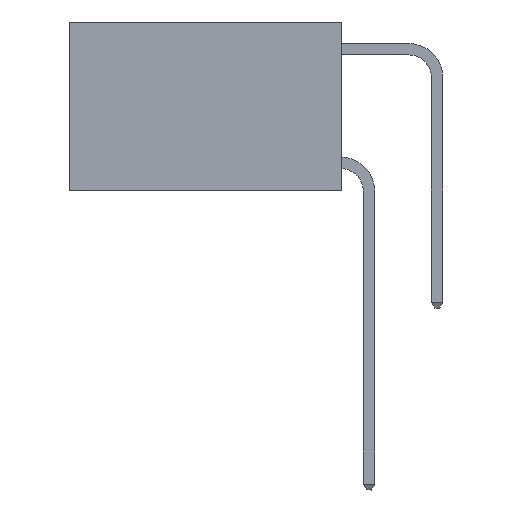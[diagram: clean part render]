
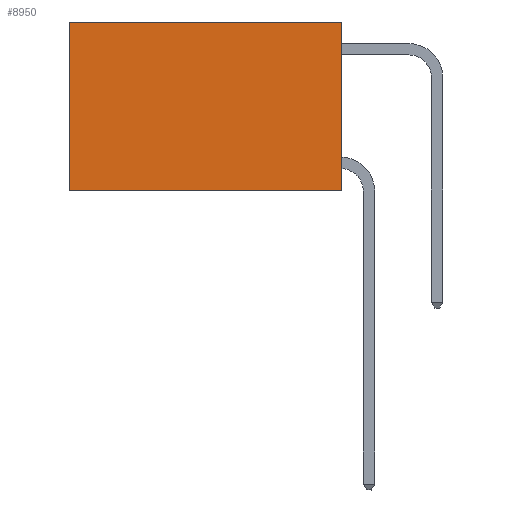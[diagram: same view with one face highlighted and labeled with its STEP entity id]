
A CAD part, left-side view. The second image highlights one B-rep face of the part: STEP entity #8950.
In plain terms, the highlighted planar face has unit normal (-1, 0, 0).
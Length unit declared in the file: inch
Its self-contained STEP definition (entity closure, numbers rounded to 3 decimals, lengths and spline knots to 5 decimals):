
#81 = CARTESIAN_POINT ( 'NONE',  ( 0.2625, 0.6, 0. ) ) ;
#233 = DIRECTION ( 'NONE',  ( 0., 0., -1. ) ) ;
#445 = DIRECTION ( 'NONE',  ( 0., 1., 0. ) ) ;
#879 = VERTEX_POINT ( 'NONE', #8515 ) ;
#906 = DIRECTION ( 'NONE',  ( 1., 0., 0. ) ) ;
#3170 = VERTEX_POINT ( 'NONE', #13100 ) ;
#3393 = EDGE_CURVE ( 'NONE', #3170, #18591, #6022, .T. ) ;
#3597 = DIRECTION ( 'NONE',  ( 0., 1., 0. ) ) ;
#4404 = LINE ( 'NONE', #12452, #21673 ) ;
#6022 = LINE ( 'NONE', #11859, #11785 ) ;
#6331 = ORIENTED_EDGE ( 'NONE', *, *, #19138, .F. ) ;
#8094 = FACE_OUTER_BOUND ( 'NONE', #11642, .T. ) ;
#8515 = CARTESIAN_POINT ( 'NONE',  ( 0.2625, 0.6, -0.37 ) ) ;
#8950 = ADVANCED_FACE ( 'NONE', ( #8094 ), #9253, .F. ) ;
#9253 = PLANE ( 'NONE',  #16056 ) ;
#9595 = EDGE_CURVE ( 'NONE', #21135, #879, #4404, .T. ) ;
#9811 = DIRECTION ( 'NONE',  ( 0., 0., -1. ) ) ;
#10939 = CARTESIAN_POINT ( 'NONE',  ( 0.2625, 0., 0. ) ) ;
#11530 = VECTOR ( 'NONE', #233, 39.37008 ) ;
#11642 = EDGE_LOOP ( 'NONE', ( #13891, #17127, #6331, #15217 ) ) ;
#11785 = VECTOR ( 'NONE', #3597, 39.37008 ) ;
#11859 = CARTESIAN_POINT ( 'NONE',  ( 0.2625, 0., 0. ) ) ;
#12176 = VECTOR ( 'NONE', #9811, 39.37008 ) ;
#12452 = CARTESIAN_POINT ( 'NONE',  ( 0.2625, 0., -0.37 ) ) ;
#13100 = CARTESIAN_POINT ( 'NONE',  ( 0.2625, 0., 0. ) ) ;
#13182 = CARTESIAN_POINT ( 'NONE',  ( 0.2625, 0., 0. ) ) ;
#13187 = CARTESIAN_POINT ( 'NONE',  ( 0.2625, 0., -0.37 ) ) ;
#13671 = EDGE_CURVE ( 'NONE', #18591, #879, #19641, .T. ) ;
#13891 = ORIENTED_EDGE ( 'NONE', *, *, #13671, .T. ) ;
#15217 = ORIENTED_EDGE ( 'NONE', *, *, #3393, .T. ) ;
#16056 = AXIS2_PLACEMENT_3D ( 'NONE', #10939, #906, #19188 ) ;
#17127 = ORIENTED_EDGE ( 'NONE', *, *, #9595, .F. ) ;
#18591 = VERTEX_POINT ( 'NONE', #18746 ) ;
#18746 = CARTESIAN_POINT ( 'NONE',  ( 0.2625, 0.6, 0. ) ) ;
#19138 = EDGE_CURVE ( 'NONE', #3170, #21135, #21056, .T. ) ;
#19188 = DIRECTION ( 'NONE',  ( 0., 0., -1. ) ) ;
#19641 = LINE ( 'NONE', #81, #11530 ) ;
#21056 = LINE ( 'NONE', #13182, #12176 ) ;
#21135 = VERTEX_POINT ( 'NONE', #13187 ) ;
#21673 = VECTOR ( 'NONE', #445, 39.37008 ) ;
